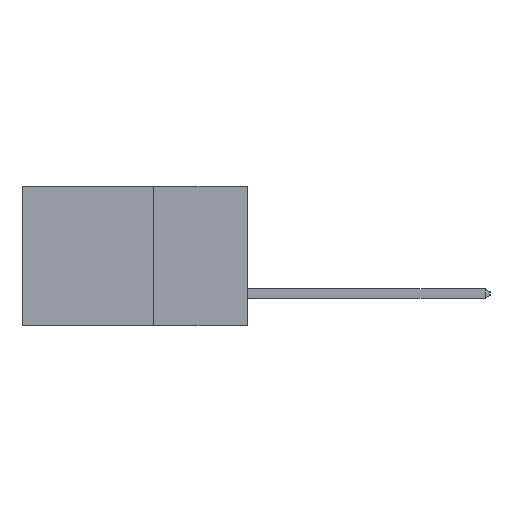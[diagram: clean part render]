
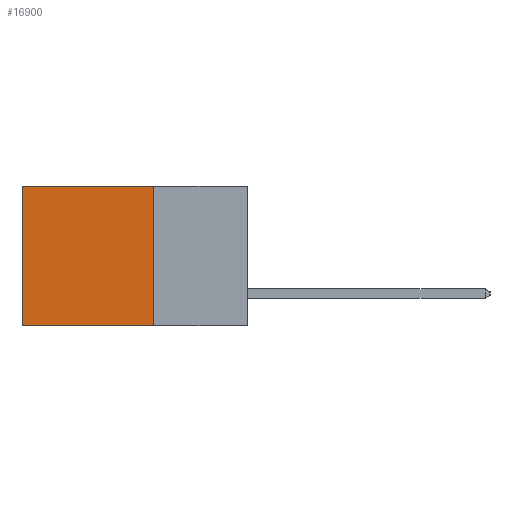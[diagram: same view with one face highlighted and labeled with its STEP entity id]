
A CAD part, left-side view. The second image highlights one B-rep face of the part: STEP entity #16900.
In plain terms, the highlighted planar face has unit normal (-1, 0, 0).
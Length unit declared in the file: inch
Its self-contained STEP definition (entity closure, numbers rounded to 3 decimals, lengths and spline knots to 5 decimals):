
#73 = DIRECTION ( 'NONE',  ( 0., 0., -1. ) ) ;
#1013 = DIRECTION ( 'NONE',  ( 0., 1., 0. ) ) ;
#2331 = DIRECTION ( 'NONE',  ( 0., 0., -1. ) ) ;
#2386 = CARTESIAN_POINT ( 'NONE',  ( 0.2615, 0.25, -0.37 ) ) ;
#2551 = VECTOR ( 'NONE', #2331, 39.37008 ) ;
#2663 = DIRECTION ( 'NONE',  ( 0., 1., 0. ) ) ;
#3098 = LINE ( 'NONE', #16438, #22942 ) ;
#3822 = VERTEX_POINT ( 'NONE', #15265 ) ;
#3960 = ORIENTED_EDGE ( 'NONE', *, *, #4937, .F. ) ;
#4025 = LINE ( 'NONE', #23121, #23816 ) ;
#4306 = ORIENTED_EDGE ( 'NONE', *, *, #11361, .F. ) ;
#4937 = EDGE_CURVE ( 'NONE', #3822, #20814, #7173, .T. ) ;
#5196 = FACE_OUTER_BOUND ( 'NONE', #19902, .T. ) ;
#6718 = CARTESIAN_POINT ( 'NONE',  ( 0.2615, 0.25, -0.37 ) ) ;
#7173 = LINE ( 'NONE', #2386, #2551 ) ;
#7426 = EDGE_CURVE ( 'NONE', #14480, #11356, #15462, .T. ) ;
#9859 = CARTESIAN_POINT ( 'NONE',  ( 0.2615, 0.6, -0.37 ) ) ;
#10609 = PLANE ( 'NONE',  #19788 ) ;
#11356 = VERTEX_POINT ( 'NONE', #15472 ) ;
#11361 = EDGE_CURVE ( 'NONE', #20814, #11356, #4025, .T. ) ;
#12540 = DIRECTION ( 'NONE',  ( 0., 0., -1. ) ) ;
#13631 = ORIENTED_EDGE ( 'NONE', *, *, #20494, .T. ) ;
#14480 = VERTEX_POINT ( 'NONE', #24361 ) ;
#14867 = VECTOR ( 'NONE', #73, 39.37008 ) ;
#15038 = ORIENTED_EDGE ( 'NONE', *, *, #7426, .T. ) ;
#15265 = CARTESIAN_POINT ( 'NONE',  ( 0.2615, 0.25, 0. ) ) ;
#15462 = LINE ( 'NONE', #9859, #14867 ) ;
#15472 = CARTESIAN_POINT ( 'NONE',  ( 0.2615, 0.6, -0.37 ) ) ;
#16438 = CARTESIAN_POINT ( 'NONE',  ( 0.2615, 0.25, 0. ) ) ;
#16900 = ADVANCED_FACE ( 'NONE', ( #5196 ), #10609, .F. ) ;
#19788 = AXIS2_PLACEMENT_3D ( 'NONE', #6718, #23924, #12540 ) ;
#19902 = EDGE_LOOP ( 'NONE', ( #15038, #4306, #3960, #13631 ) ) ;
#20494 = EDGE_CURVE ( 'NONE', #3822, #14480, #3098, .T. ) ;
#20814 = VERTEX_POINT ( 'NONE', #21066 ) ;
#21066 = CARTESIAN_POINT ( 'NONE',  ( 0.2615, 0.25, -0.37 ) ) ;
#22942 = VECTOR ( 'NONE', #1013, 39.37008 ) ;
#23121 = CARTESIAN_POINT ( 'NONE',  ( 0.2615, 0.25, -0.37 ) ) ;
#23816 = VECTOR ( 'NONE', #2663, 39.37008 ) ;
#23924 = DIRECTION ( 'NONE',  ( 1., 0., 0. ) ) ;
#24361 = CARTESIAN_POINT ( 'NONE',  ( 0.2615, 0.6, 0. ) ) ;
